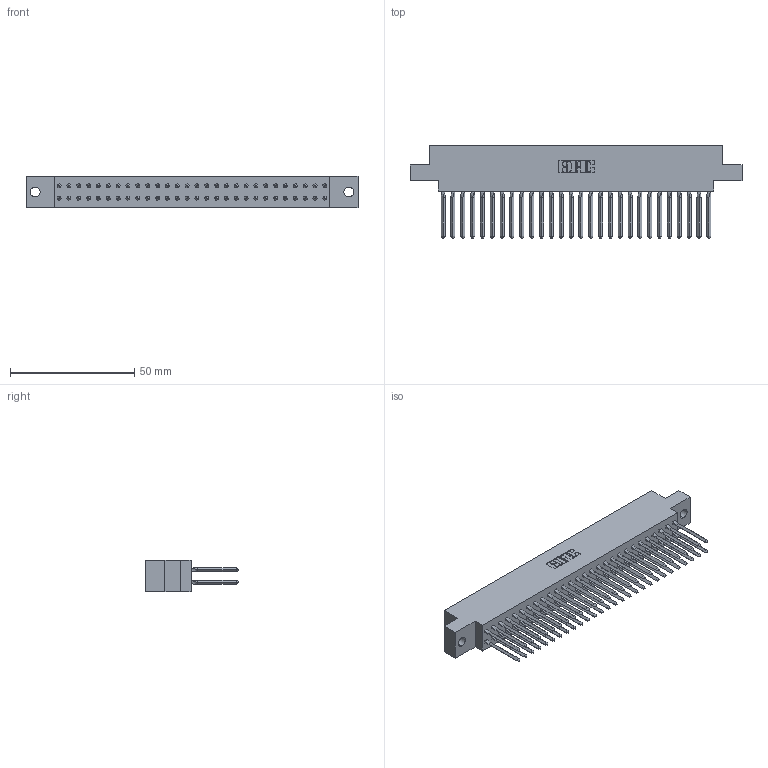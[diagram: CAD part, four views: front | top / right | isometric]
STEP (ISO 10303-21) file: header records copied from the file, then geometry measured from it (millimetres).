
FILE_DESCRIPTION (( 'STEP AP203' ), '1' );
FILE_NAME ('317-056-542-804.STEP', '2020-02-28T04:20:05', ( '' ), ( '' ), 'SwSTEP 2.0', 'SolidWorks 2016', '' );
FILE_SCHEMA (( 'CONFIG_CONTROL_DESIGN' ));
Length unit declared in the file: inch
Products named in the file (3): 317 Part_.156 Dia - TH; 317-290-003_542; 317-056-542-804
Assembly tree (57 placements, depth 2):
  317-056-542-804
    317 Part_.156 Dia - TH
    317-290-003_542  x56
Bounding box: 133.65 x 37.34 x 12.7 mm (x, y, z)
Volume: 21355.2 mm3; surface area: 29064.3 mm2
Topology: 57 solids, 57 shells, 3294 faces, 9235 edges, 5894 vertices
Faces by surface type: plane 2634, cylinder 436, bspline 224
Entity records: 41447 total; most frequent: CARTESIAN_POINT 7477, ORIENTED_EDGE 7140, DIRECTION 6030, EDGE_CURVE 3570, LINE 3400, VECTOR 3400, VERTEX_POINT 2374, AXIS2_PLACEMENT_3D 1315
